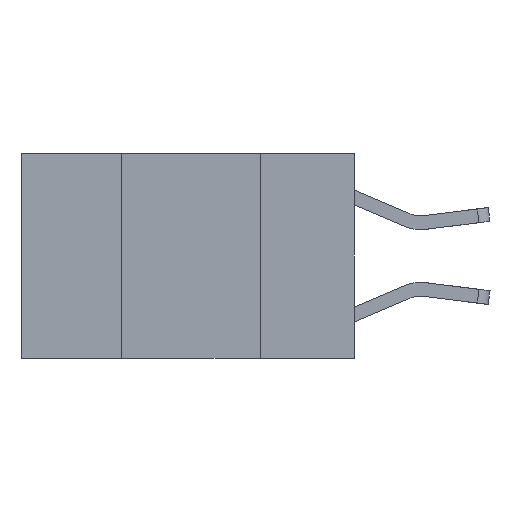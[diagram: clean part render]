
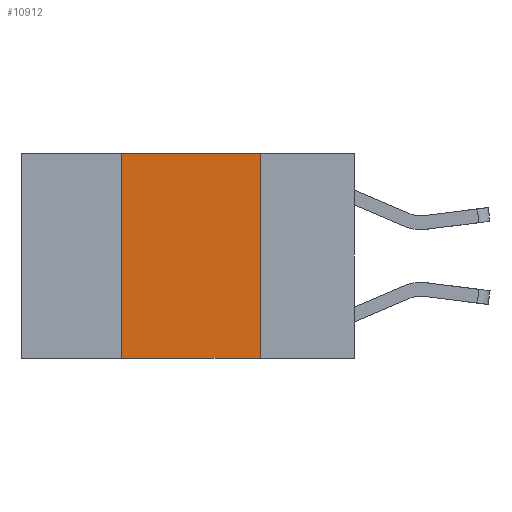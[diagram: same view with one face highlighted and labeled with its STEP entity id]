
A CAD part, left-side view. The second image highlights one B-rep face of the part: STEP entity #10912.
In plain terms, the highlighted planar face has unit normal (-1, 0, 0).
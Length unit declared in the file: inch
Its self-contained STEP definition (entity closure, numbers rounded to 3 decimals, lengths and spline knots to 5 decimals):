
#326 = VECTOR ( 'NONE', #3487, 39.37008 ) ;
#711 = PLANE ( 'NONE',  #9791 ) ;
#747 = DIRECTION ( 'NONE',  ( 0., 0., -1. ) ) ;
#1483 = CARTESIAN_POINT ( 'NONE',  ( 0., 0.42, 0. ) ) ;
#2167 = EDGE_CURVE ( 'NONE', #7610, #3259, #7227, .T. ) ;
#2180 = VECTOR ( 'NONE', #2904, 39.37008 ) ;
#2548 = CARTESIAN_POINT ( 'NONE',  ( 0., 0.6, -0.37 ) ) ;
#2873 = CARTESIAN_POINT ( 'NONE',  ( 0., 0.17, 0. ) ) ;
#2904 = DIRECTION ( 'NONE',  ( 0., 0., -1. ) ) ;
#3075 = CARTESIAN_POINT ( 'NONE',  ( 0., 0.42, 0. ) ) ;
#3259 = VERTEX_POINT ( 'NONE', #6558 ) ;
#3487 = DIRECTION ( 'NONE',  ( 0., -1., 0. ) ) ;
#3958 = ORIENTED_EDGE ( 'NONE', *, *, #2167, .F. ) ;
#4346 = DIRECTION ( 'NONE',  ( 0., -1., 0. ) ) ;
#4412 = CARTESIAN_POINT ( 'NONE',  ( 0., 0.17, 0. ) ) ;
#4491 = VECTOR ( 'NONE', #8102, 39.37008 ) ;
#4924 = VERTEX_POINT ( 'NONE', #3075 ) ;
#4936 = EDGE_LOOP ( 'NONE', ( #3958, #6497, #9006, #11440 ) ) ;
#5127 = EDGE_CURVE ( 'NONE', #4924, #7610, #7732, .T. ) ;
#5374 = LINE ( 'NONE', #2548, #326 ) ;
#6441 = DIRECTION ( 'NONE',  ( 1., 0., 0. ) ) ;
#6497 = ORIENTED_EDGE ( 'NONE', *, *, #5127, .F. ) ;
#6558 = CARTESIAN_POINT ( 'NONE',  ( 0., 0.17, -0.37 ) ) ;
#6894 = FACE_OUTER_BOUND ( 'NONE', #4936, .T. ) ;
#7227 = LINE ( 'NONE', #2873, #2180 ) ;
#7610 = VERTEX_POINT ( 'NONE', #4412 ) ;
#7732 = LINE ( 'NONE', #10916, #10190 ) ;
#8005 = VERTEX_POINT ( 'NONE', #10608 ) ;
#8102 = DIRECTION ( 'NONE',  ( 0., 0., 1. ) ) ;
#9006 = ORIENTED_EDGE ( 'NONE', *, *, #10001, .F. ) ;
#9791 = AXIS2_PLACEMENT_3D ( 'NONE', #12008, #6441, #747 ) ;
#10001 = EDGE_CURVE ( 'NONE', #8005, #4924, #11676, .T. ) ;
#10190 = VECTOR ( 'NONE', #4346, 39.37008 ) ;
#10608 = CARTESIAN_POINT ( 'NONE',  ( 0., 0.42, -0.37 ) ) ;
#10819 = EDGE_CURVE ( 'NONE', #8005, #3259, #5374, .T. ) ;
#10912 = ADVANCED_FACE ( 'NONE', ( #6894 ), #711, .F. ) ;
#10916 = CARTESIAN_POINT ( 'NONE',  ( 0., 0.6, 0. ) ) ;
#11440 = ORIENTED_EDGE ( 'NONE', *, *, #10819, .T. ) ;
#11676 = LINE ( 'NONE', #1483, #4491 ) ;
#12008 = CARTESIAN_POINT ( 'NONE',  ( 0., 0.6, 0. ) ) ;
